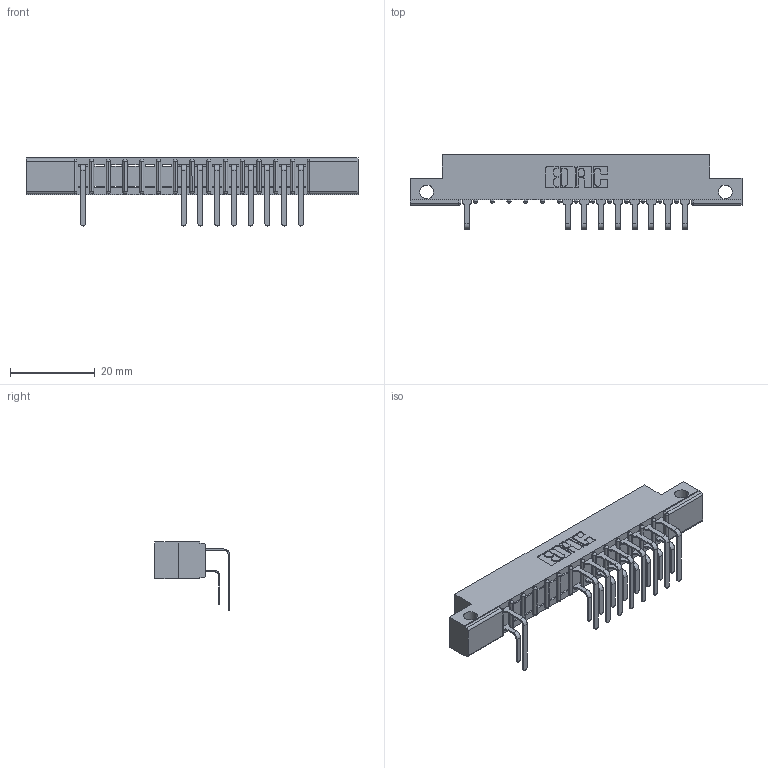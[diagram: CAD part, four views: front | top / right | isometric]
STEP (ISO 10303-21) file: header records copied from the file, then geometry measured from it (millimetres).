
FILE_DESCRIPTION (( 'STEP AP203' ), '1' );
FILE_NAME ('357-014-559-112.STEP', '2018-08-07T23:42:24', ( '' ), ( '' ), 'SwSTEP 2.0', 'SolidWorks 2016', '' );
FILE_SCHEMA (( 'CONFIG_CONTROL_DESIGN' ));
Length unit declared in the file: inch
Products named in the file (4): 307 Part_.128 Dia Side Mounting Holes; 307-290-001_558 559 - 1 (Single); 307-290-001_559 - 2 (Single); 357-014-559-112
Assembly tree (19 placements, depth 2):
  357-014-559-112
    307 Part_.128 Dia Side Mounting Holes
    307-290-001_558 559 - 1 (Single)  x9
    307-290-001_559 - 2 (Single)  x9
Bounding box: 78.49 x 17.69 x 16.08 mm (x, y, z)
Volume: 5009.1 mm3; surface area: 7976.5 mm2
Topology: 19 solids, 19 shells, 1133 faces, 3199 edges, 2066 vertices
Faces by surface type: plane 724, cylinder 379, sphere 30
Entity records: 17031 total; most frequent: CARTESIAN_POINT 2838, ORIENTED_EDGE 2818, DIRECTION 2781, EDGE_CURVE 1409, LINE 1067, VECTOR 1067, VERTEX_POINT 914, AXIS2_PLACEMENT_3D 857
